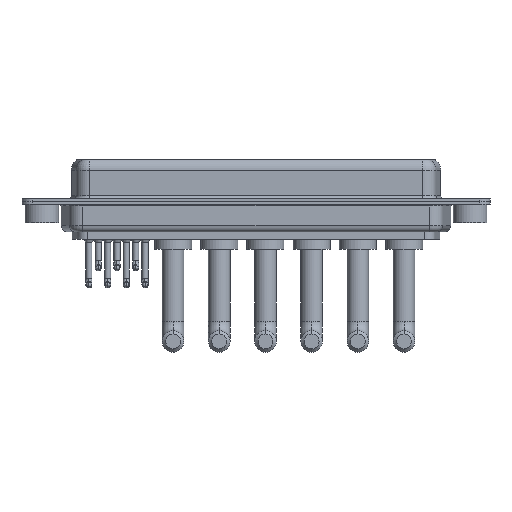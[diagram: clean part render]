
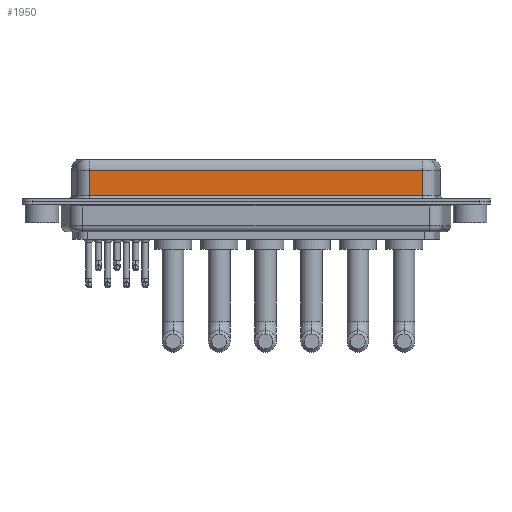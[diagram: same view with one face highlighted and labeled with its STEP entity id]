
A CAD part, front view. The second image highlights one B-rep face of the part: STEP entity #1950.
In plain terms, the highlighted planar face has unit normal (0, -1, 0).
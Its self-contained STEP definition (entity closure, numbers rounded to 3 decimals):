
#1147 = FACE_OUTER_BOUND ( 'NONE', #7253, .T. ) ;
#1729 = EDGE_CURVE ( 'NONE', #2285, #9983, #8606, .T. ) ;
#1784 = ORIENTED_EDGE ( 'NONE', *, *, #9211, .T. ) ;
#1950 = ADVANCED_FACE ( 'NONE', ( #1147 ), #3936, .F. ) ;
#2230 = CARTESIAN_POINT ( 'NONE',  ( 56.462, -3.95, 0.9 ) ) ;
#2285 = VERTEX_POINT ( 'NONE', #6602 ) ;
#2546 = DIRECTION ( 'NONE',  ( 0., 1., 0. ) ) ;
#3936 = PLANE ( 'NONE',  #5121 ) ;
#4244 = VECTOR ( 'NONE', #7837, 1000. ) ;
#4278 = CARTESIAN_POINT ( 'NONE',  ( 56.462, -3.95, 4.65 ) ) ;
#4773 = DIRECTION ( 'NONE',  ( 0., 0., -1. ) ) ;
#4812 = EDGE_CURVE ( 'NONE', #9107, #5324, #9127, .T. ) ;
#5121 = AXIS2_PLACEMENT_3D ( 'NONE', #15291, #2546, #8199 ) ;
#5324 = VERTEX_POINT ( 'NONE', #5959 ) ;
#5959 = CARTESIAN_POINT ( 'NONE',  ( 56.462, -3.95, 0.9 ) ) ;
#6353 = CARTESIAN_POINT ( 'NONE',  ( 7.038, -3.95, 6.4 ) ) ;
#6405 = DIRECTION ( 'NONE',  ( 1., 0., 0. ) ) ;
#6602 = CARTESIAN_POINT ( 'NONE',  ( 7.038, -3.95, 4.65 ) ) ;
#6850 = EDGE_CURVE ( 'NONE', #9107, #2285, #17814, .T. ) ;
#7253 = EDGE_LOOP ( 'NONE', ( #13885, #13871, #17167, #1784 ) ) ;
#7727 = VECTOR ( 'NONE', #4773, 1000. ) ;
#7837 = DIRECTION ( 'NONE',  ( -1., 0., 0. ) ) ;
#8199 = DIRECTION ( 'NONE',  ( 0., 0., 1. ) ) ;
#8606 = LINE ( 'NONE', #6353, #14048 ) ;
#9039 = CARTESIAN_POINT ( 'NONE',  ( 7.038, -3.95, 0.9 ) ) ;
#9107 = VERTEX_POINT ( 'NONE', #4278 ) ;
#9127 = LINE ( 'NONE', #14793, #7727 ) ;
#9211 = EDGE_CURVE ( 'NONE', #9983, #5324, #14685, .T. ) ;
#9983 = VERTEX_POINT ( 'NONE', #9039 ) ;
#13699 = CARTESIAN_POINT ( 'NONE',  ( 56.462, -3.95, 4.65 ) ) ;
#13871 = ORIENTED_EDGE ( 'NONE', *, *, #6850, .T. ) ;
#13885 = ORIENTED_EDGE ( 'NONE', *, *, #4812, .F. ) ;
#14048 = VECTOR ( 'NONE', #15883, 1000. ) ;
#14098 = VECTOR ( 'NONE', #6405, 1000. ) ;
#14685 = LINE ( 'NONE', #2230, #14098 ) ;
#14793 = CARTESIAN_POINT ( 'NONE',  ( 56.462, -3.95, 6.4 ) ) ;
#15291 = CARTESIAN_POINT ( 'NONE',  ( 56.462, -3.95, 6.4 ) ) ;
#15883 = DIRECTION ( 'NONE',  ( 0., 0., -1. ) ) ;
#17167 = ORIENTED_EDGE ( 'NONE', *, *, #1729, .T. ) ;
#17814 = LINE ( 'NONE', #13699, #4244 ) ;
